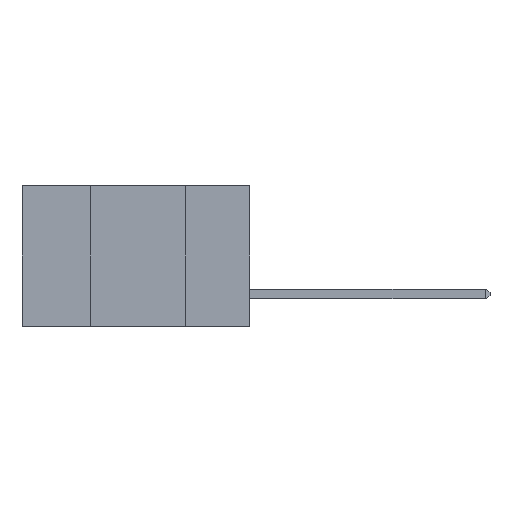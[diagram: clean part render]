
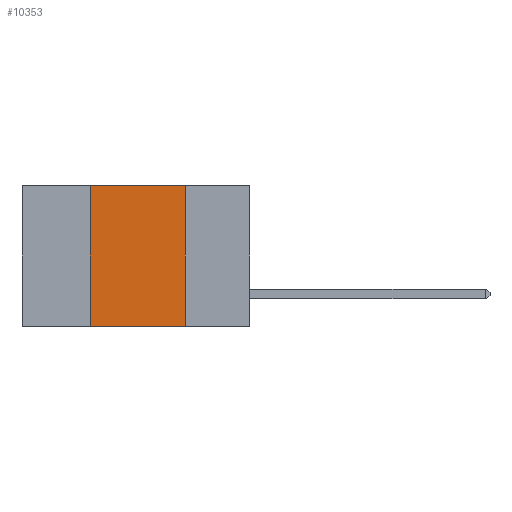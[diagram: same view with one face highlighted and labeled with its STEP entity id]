
A CAD part, left-side view. The second image highlights one B-rep face of the part: STEP entity #10353.
In plain terms, the highlighted planar face has unit normal (-1, 0, 0).
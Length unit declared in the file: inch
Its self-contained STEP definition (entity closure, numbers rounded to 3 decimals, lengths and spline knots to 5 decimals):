
#433 = LINE ( 'NONE', #763, #15479 ) ;
#744 = EDGE_LOOP ( 'NONE', ( #15395, #8787, #1338, #9247 ) ) ;
#763 = CARTESIAN_POINT ( 'NONE',  ( 0., 0.6, 0. ) ) ;
#847 = CARTESIAN_POINT ( 'NONE',  ( 0., 0.6, 0. ) ) ;
#1338 = ORIENTED_EDGE ( 'NONE', *, *, #4797, .F. ) ;
#2385 = DIRECTION ( 'NONE',  ( 1., 0., 0. ) ) ;
#3719 = CARTESIAN_POINT ( 'NONE',  ( 0., 0.17, -0.37 ) ) ;
#3805 = VECTOR ( 'NONE', #17560, 39.37008 ) ;
#4797 = EDGE_CURVE ( 'NONE', #8488, #7170, #8840, .T. ) ;
#4910 = VECTOR ( 'NONE', #17614, 39.37008 ) ;
#6434 = AXIS2_PLACEMENT_3D ( 'NONE', #847, #2385, #12570 ) ;
#6536 = LINE ( 'NONE', #12168, #13679 ) ;
#7170 = VERTEX_POINT ( 'NONE', #18513 ) ;
#8488 = VERTEX_POINT ( 'NONE', #14256 ) ;
#8787 = ORIENTED_EDGE ( 'NONE', *, *, #16153, .F. ) ;
#8840 = LINE ( 'NONE', #10560, #4910 ) ;
#9247 = ORIENTED_EDGE ( 'NONE', *, *, #15363, .T. ) ;
#10353 = ADVANCED_FACE ( 'NONE', ( #17422 ), #11166, .F. ) ;
#10560 = CARTESIAN_POINT ( 'NONE',  ( 0., 0.42, 0. ) ) ;
#11166 = PLANE ( 'NONE',  #6434 ) ;
#11956 = LINE ( 'NONE', #16163, #3805 ) ;
#12168 = CARTESIAN_POINT ( 'NONE',  ( 0., 0.17, 0. ) ) ;
#12484 = DIRECTION ( 'NONE',  ( 0., -1., 0. ) ) ;
#12570 = DIRECTION ( 'NONE',  ( 0., 0., -1. ) ) ;
#13580 = DIRECTION ( 'NONE',  ( 0., 0., -1. ) ) ;
#13679 = VECTOR ( 'NONE', #13580, 39.37008 ) ;
#14256 = CARTESIAN_POINT ( 'NONE',  ( 0., 0.42, -0.37 ) ) ;
#14375 = VERTEX_POINT ( 'NONE', #3719 ) ;
#15363 = EDGE_CURVE ( 'NONE', #8488, #14375, #11956, .T. ) ;
#15395 = ORIENTED_EDGE ( 'NONE', *, *, #16647, .F. ) ;
#15479 = VECTOR ( 'NONE', #12484, 39.37008 ) ;
#16153 = EDGE_CURVE ( 'NONE', #7170, #16922, #433, .T. ) ;
#16163 = CARTESIAN_POINT ( 'NONE',  ( 0., 0.6, -0.37 ) ) ;
#16647 = EDGE_CURVE ( 'NONE', #16922, #14375, #6536, .T. ) ;
#16922 = VERTEX_POINT ( 'NONE', #18418 ) ;
#17422 = FACE_OUTER_BOUND ( 'NONE', #744, .T. ) ;
#17560 = DIRECTION ( 'NONE',  ( 0., -1., 0. ) ) ;
#17614 = DIRECTION ( 'NONE',  ( 0., 0., 1. ) ) ;
#18418 = CARTESIAN_POINT ( 'NONE',  ( 0., 0.17, 0. ) ) ;
#18513 = CARTESIAN_POINT ( 'NONE',  ( 0., 0.42, 0. ) ) ;
